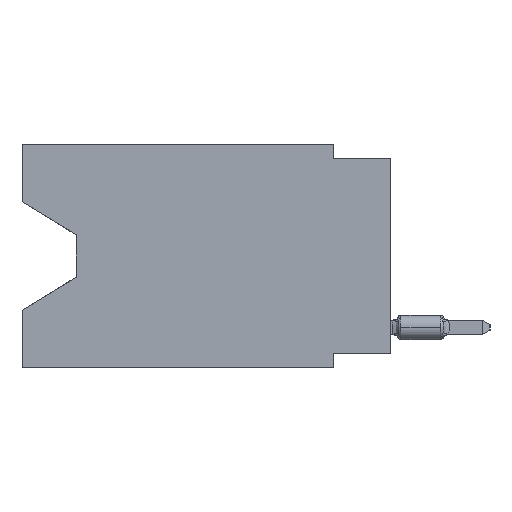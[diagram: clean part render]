
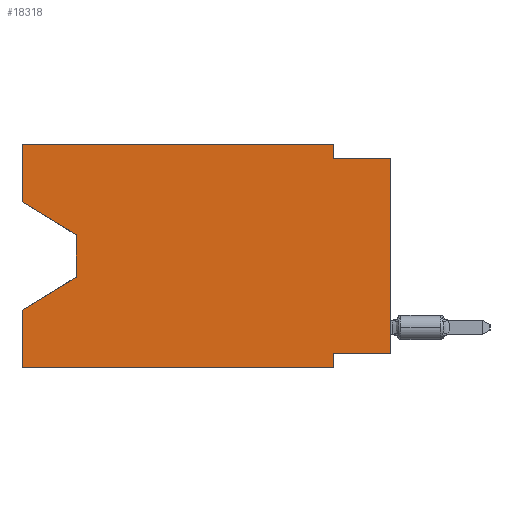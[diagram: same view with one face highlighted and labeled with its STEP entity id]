
A CAD part, left-side view. The second image highlights one B-rep face of the part: STEP entity #18318.
In plain terms, the highlighted planar face has unit normal (-1, 0, 0).
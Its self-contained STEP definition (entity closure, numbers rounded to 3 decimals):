
#43 = CARTESIAN_POINT ( 'NONE',  ( 0., 16.383, -9.906 ) ) ;
#396 = VERTEX_POINT ( 'NONE', #9386 ) ;
#783 = VERTEX_POINT ( 'NONE', #52100 ) ;
#921 = VECTOR ( 'NONE', #50453, 1000. ) ;
#1262 = CARTESIAN_POINT ( 'NONE',  ( 0., 0., 0. ) ) ;
#1901 = ORIENTED_EDGE ( 'NONE', *, *, #9110, .T. ) ;
#2307 = VERTEX_POINT ( 'NONE', #46058 ) ;
#2760 = CARTESIAN_POINT ( 'NONE',  ( 0., 16.383, -7.36 ) ) ;
#4124 = LINE ( 'NONE', #4391, #22183 ) ;
#4391 = CARTESIAN_POINT ( 'NONE',  ( 0., 0., -0.635 ) ) ;
#4545 = ORIENTED_EDGE ( 'NONE', *, *, #23520, .F. ) ;
#5159 = ORIENTED_EDGE ( 'NONE', *, *, #8432, .F. ) ;
#5571 = VERTEX_POINT ( 'NONE', #32842 ) ;
#5629 = CARTESIAN_POINT ( 'NONE',  ( 0., 0., -9.271 ) ) ;
#5704 = LINE ( 'NONE', #38742, #17753 ) ;
#6242 = DIRECTION ( 'NONE',  ( 0., 0., 1. ) ) ;
#6743 = CARTESIAN_POINT ( 'NONE',  ( 0., 2.54, -9.906 ) ) ;
#7866 = LINE ( 'NONE', #43, #16896 ) ;
#8432 = EDGE_CURVE ( 'NONE', #48052, #396, #17730, .T. ) ;
#9067 = DIRECTION ( 'NONE',  ( 0., 0., -1. ) ) ;
#9110 = EDGE_CURVE ( 'NONE', #11591, #46311, #22273, .T. ) ;
#9154 = CARTESIAN_POINT ( 'NONE',  ( 0., 13.97, -5.893 ) ) ;
#9386 = CARTESIAN_POINT ( 'NONE',  ( 0., 2.54, -9.906 ) ) ;
#10890 = EDGE_CURVE ( 'NONE', #5571, #26069, #14645, .T. ) ;
#11548 = CARTESIAN_POINT ( 'NONE',  ( 0., 16.383, 0. ) ) ;
#11591 = VERTEX_POINT ( 'NONE', #5629 ) ;
#11644 = EDGE_LOOP ( 'NONE', ( #37571, #19612, #42911, #24534, #48634, #5159, #50824, #1901, #17872, #21160, #43850, #4545 ) ) ;
#14645 = LINE ( 'NONE', #11548, #15962 ) ;
#15962 = VECTOR ( 'NONE', #6242, 1000. ) ;
#16557 = DIRECTION ( 'NONE',  ( 0., 0., 1. ) ) ;
#16896 = VECTOR ( 'NONE', #20494, 1000. ) ;
#17730 = LINE ( 'NONE', #6743, #48820 ) ;
#17753 = VECTOR ( 'NONE', #31174, 1000. ) ;
#17872 = ORIENTED_EDGE ( 'NONE', *, *, #31408, .F. ) ;
#18318 = ADVANCED_FACE ( 'NONE', ( #42269 ), #41987, .F. ) ;
#19010 = DIRECTION ( 'NONE',  ( 0., 1., 0. ) ) ;
#19225 = VECTOR ( 'NONE', #31980, 1000. ) ;
#19612 = ORIENTED_EDGE ( 'NONE', *, *, #36596, .T. ) ;
#20145 = VECTOR ( 'NONE', #19010, 1000. ) ;
#20494 = DIRECTION ( 'NONE',  ( 0., -1., 0. ) ) ;
#20525 = LINE ( 'NONE', #54599, #19225 ) ;
#20746 = CARTESIAN_POINT ( 'NONE',  ( 0., 16.383, 0. ) ) ;
#20752 = LINE ( 'NONE', #54822, #44994 ) ;
#21160 = ORIENTED_EDGE ( 'NONE', *, *, #27544, .F. ) ;
#21218 = LINE ( 'NONE', #9154, #25763 ) ;
#22183 = VECTOR ( 'NONE', #38825, 1000. ) ;
#22273 = LINE ( 'NONE', #1262, #42632 ) ;
#23520 = EDGE_CURVE ( 'NONE', #28560, #783, #20752, .T. ) ;
#23746 = LINE ( 'NONE', #27383, #20145 ) ;
#23851 = DIRECTION ( 'NONE',  ( 0., 0., -1. ) ) ;
#24534 = ORIENTED_EDGE ( 'NONE', *, *, #10890, .F. ) ;
#24884 = VERTEX_POINT ( 'NONE', #31873 ) ;
#25763 = VECTOR ( 'NONE', #30425, 1000. ) ;
#26069 = VERTEX_POINT ( 'NONE', #2760 ) ;
#27155 = CARTESIAN_POINT ( 'NONE',  ( 0., 13.97, -4.013 ) ) ;
#27383 = CARTESIAN_POINT ( 'NONE',  ( 0., 0., -9.271 ) ) ;
#27544 = EDGE_CURVE ( 'NONE', #45158, #24884, #38461, .T. ) ;
#28560 = VERTEX_POINT ( 'NONE', #31580 ) ;
#28993 = VECTOR ( 'NONE', #9067, 1000. ) ;
#29503 = LINE ( 'NONE', #45706, #921 ) ;
#30195 = CARTESIAN_POINT ( 'NONE',  ( 0., 2.54, 0. ) ) ;
#30425 = DIRECTION ( 'NONE',  ( 0., 0.855, -0.519 ) ) ;
#30676 = EDGE_CURVE ( 'NONE', #28560, #51746, #5704, .T. ) ;
#31174 = DIRECTION ( 'NONE',  ( 0., -0.855, -0.519 ) ) ;
#31408 = EDGE_CURVE ( 'NONE', #24884, #46311, #4124, .T. ) ;
#31439 = EDGE_CURVE ( 'NONE', #2307, #26069, #21218, .T. ) ;
#31580 = CARTESIAN_POINT ( 'NONE',  ( 0., 16.383, -2.546 ) ) ;
#31873 = CARTESIAN_POINT ( 'NONE',  ( 0., 2.54, -0.635 ) ) ;
#31980 = DIRECTION ( 'NONE',  ( 0., 0., -1. ) ) ;
#32842 = CARTESIAN_POINT ( 'NONE',  ( 0., 16.383, -9.906 ) ) ;
#33880 = DIRECTION ( 'NONE',  ( 0., 0., -1. ) ) ;
#33956 = EDGE_CURVE ( 'NONE', #5571, #396, #7866, .T. ) ;
#36596 = EDGE_CURVE ( 'NONE', #51746, #2307, #20525, .T. ) ;
#36769 = EDGE_CURVE ( 'NONE', #11591, #48052, #23746, .T. ) ;
#37571 = ORIENTED_EDGE ( 'NONE', *, *, #30676, .T. ) ;
#38461 = LINE ( 'NONE', #55210, #28993 ) ;
#38742 = CARTESIAN_POINT ( 'NONE',  ( 0., 16.383, -2.546 ) ) ;
#38825 = DIRECTION ( 'NONE',  ( 0., -1., 0. ) ) ;
#39418 = CARTESIAN_POINT ( 'NONE',  ( 0., 2.54, -9.271 ) ) ;
#41987 = PLANE ( 'NONE',  #52424 ) ;
#42269 = FACE_OUTER_BOUND ( 'NONE', #11644, .T. ) ;
#42632 = VECTOR ( 'NONE', #43489, 1000. ) ;
#42911 = ORIENTED_EDGE ( 'NONE', *, *, #31439, .T. ) ;
#43489 = DIRECTION ( 'NONE',  ( 0., 0., 1. ) ) ;
#43850 = ORIENTED_EDGE ( 'NONE', *, *, #49763, .F. ) ;
#44994 = VECTOR ( 'NONE', #16557, 1000. ) ;
#45158 = VERTEX_POINT ( 'NONE', #30195 ) ;
#45706 = CARTESIAN_POINT ( 'NONE',  ( 0., 16.383, 0. ) ) ;
#46058 = CARTESIAN_POINT ( 'NONE',  ( 0., 13.97, -5.893 ) ) ;
#46311 = VERTEX_POINT ( 'NONE', #48174 ) ;
#48052 = VERTEX_POINT ( 'NONE', #39418 ) ;
#48174 = CARTESIAN_POINT ( 'NONE',  ( 0., 0., -0.635 ) ) ;
#48634 = ORIENTED_EDGE ( 'NONE', *, *, #33956, .T. ) ;
#48820 = VECTOR ( 'NONE', #23851, 1000. ) ;
#49763 = EDGE_CURVE ( 'NONE', #783, #45158, #29503, .T. ) ;
#50453 = DIRECTION ( 'NONE',  ( 0., -1., 0. ) ) ;
#50824 = ORIENTED_EDGE ( 'NONE', *, *, #36769, .F. ) ;
#50891 = DIRECTION ( 'NONE',  ( 1., 0., 0. ) ) ;
#51746 = VERTEX_POINT ( 'NONE', #27155 ) ;
#52100 = CARTESIAN_POINT ( 'NONE',  ( 0., 16.383, 0. ) ) ;
#52424 = AXIS2_PLACEMENT_3D ( 'NONE', #20746, #50891, #33880 ) ;
#54599 = CARTESIAN_POINT ( 'NONE',  ( 0., 13.97, -4.013 ) ) ;
#54822 = CARTESIAN_POINT ( 'NONE',  ( 0., 16.383, 0. ) ) ;
#55210 = CARTESIAN_POINT ( 'NONE',  ( 0., 2.54, 0. ) ) ;
